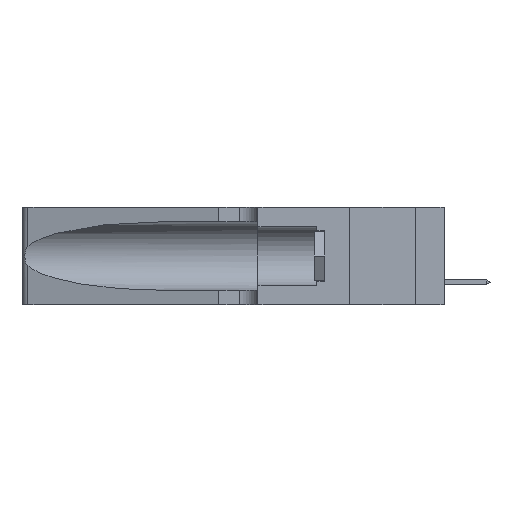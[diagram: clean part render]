
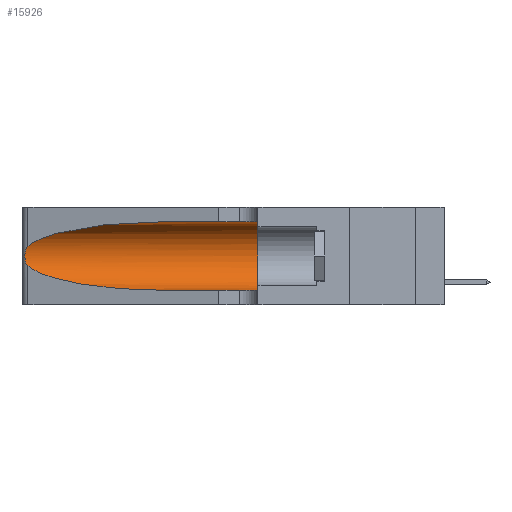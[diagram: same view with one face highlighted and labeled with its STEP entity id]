
A CAD part, left-side view. The second image highlights one B-rep face of the part: STEP entity #15926.
In plain terms, the highlighted cylindrical face has radius 3.308 mm (diameter 6.617 mm), a partial arc.
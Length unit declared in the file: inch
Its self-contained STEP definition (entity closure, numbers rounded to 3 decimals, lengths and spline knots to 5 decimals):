
#88 = CARTESIAN_POINT ( 'NONE',  ( 0.25487, 1.22718, 0.22369 ) ) ;
#142 = CARTESIAN_POINT ( 'NONE',  ( 0.25487, 1.22718, 0.22369 ) ) ;
#237 = CARTESIAN_POINT ( 'NONE',  ( 0.25854, 1.2359, 0.20912 ) ) ;
#312 = CARTESIAN_POINT ( 'NONE',  ( 0.25487, 1.22718, 0.22369 ) ) ;
#527 = CARTESIAN_POINT ( 'NONE',  ( 0.18966, 0.96281, 0.05475 ) ) ;
#576 = DIRECTION ( 'NONE',  ( 0., 0., -1. ) ) ;
#703 = VERTEX_POINT ( 'NONE', #16997 ) ;
#1011 = CARTESIAN_POINT ( 'NONE',  ( 0.1305, 0.35, 0.185 ) ) ;
#1067 = ORIENTED_EDGE ( 'NONE', *, *, #16218, .T. ) ;
#1242 = B_SPLINE_CURVE_WITH_KNOTS ( 'NONE', 3,
 ( #312, #6935, #6656, #5045, #237, #13346, #3399, #16834, #8630, #11989, #6796, #20068, #18690, #10314 ),
 .UNSPECIFIED., .F., .F.,
 ( 4, 2, 2, 2, 2, 2, 4 ),
 ( 0., 0.00027, 0.00053, 0.00107, 0.0016, 0.00187, 0.00214 ),
 .UNSPECIFIED. ) ;
#1402 = ORIENTED_EDGE ( 'NONE', *, *, #5150, .T. ) ;
#1642 = CARTESIAN_POINT ( 'NONE',  ( 0.2373, 1.15595, 0.28018 ) ) ;
#1899 = CARTESIAN_POINT ( 'NONE',  ( 0.25487, 1.22718, 0.14631 ) ) ;
#2563 = VECTOR ( 'NONE', #11613, 39.37008 ) ;
#3113 = CARTESIAN_POINT ( 'NONE',  ( 0.18966, 0.96281, 0.31525 ) ) ;
#3399 = CARTESIAN_POINT ( 'NONE',  ( 0.26075, 1.23896, 0.19203 ) ) ;
#4764 = VERTEX_POINT ( 'NONE', #5331 ) ;
#5045 = CARTESIAN_POINT ( 'NONE',  ( 0.25787, 1.23484, 0.2124 ) ) ;
#5150 = EDGE_CURVE ( 'NONE', #12302, #703, #18276, .T. ) ;
#5331 = CARTESIAN_POINT ( 'NONE',  ( 0.1305, 0.72297, 0.31525 ) ) ;
#5946 = EDGE_LOOP ( 'NONE', ( #1067, #15056, #21410, #1402, #20583, #12580 ) ) ;
#6241 = CARTESIAN_POINT ( 'NONE',  ( 0.1305, 0.72297, 0.31525 ) ) ;
#6656 = CARTESIAN_POINT ( 'NONE',  ( 0.25639, 1.23184, 0.21858 ) ) ;
#6796 = CARTESIAN_POINT ( 'NONE',  ( 0.25789, 1.23486, 0.15765 ) ) ;
#6935 = CARTESIAN_POINT ( 'NONE',  ( 0.25555, 1.22994, 0.2215 ) ) ;
#7349 = DIRECTION ( 'NONE',  ( 0., -1., 0. ) ) ;
#7574 = DIRECTION ( 'NONE',  ( 0., 1., 0. ) ) ;
#8630 = CARTESIAN_POINT ( 'NONE',  ( 0.26017, 1.23833, 0.17102 ) ) ;
#9499 = EDGE_CURVE ( 'NONE', #4764, #20645, #19708, .T. ) ;
#10314 = CARTESIAN_POINT ( 'NONE',  ( 0.25487, 1.22718, 0.14631 ) ) ;
#10537 = EDGE_CURVE ( 'NONE', #16110, #12302, #18402, .T. ) ;
#11613 = DIRECTION ( 'NONE',  ( 0., -1., 0. ) ) ;
#11989 = CARTESIAN_POINT ( 'NONE',  ( 0.25856, 1.23593, 0.16098 ) ) ;
#12199 = CARTESIAN_POINT ( 'NONE',  ( 0.1305, 0.72297, 0.05475 ) ) ;
#12302 = VERTEX_POINT ( 'NONE', #18582 ) ;
#12580 = ORIENTED_EDGE ( 'NONE', *, *, #9499, .F. ) ;
#12728 = CYLINDRICAL_SURFACE ( 'NONE', #15548, 0.13025 ) ;
#13346 = CARTESIAN_POINT ( 'NONE',  ( 0.26018, 1.23835, 0.19895 ) ) ;
#13550 = VERTEX_POINT ( 'NONE', #142 ) ;
#13698 = CARTESIAN_POINT ( 'NONE',  ( 0.2373, 1.15595, 0.08982 ) ) ;
#14036 = CARTESIAN_POINT ( 'NONE',  ( 0.1305, 0.35, 0.31525 ) ) ;
#14186 = CIRCLE ( 'NONE', #18389, 0.13025 ) ;
#14517 = EDGE_CURVE ( 'NONE', #13550, #16110, #1242, .T. ) ;
#15056 = ORIENTED_EDGE ( 'NONE', *, *, #14517, .T. ) ;
#15089 = FACE_OUTER_BOUND ( 'NONE', #5946, .T. ) ;
#15548 = AXIS2_PLACEMENT_3D ( 'NONE', #18931, #7349, #576 ) ;
#15926 = ADVANCED_FACE ( 'NONE', ( #15089 ), #12728, .F. ) ;
#15973 = CARTESIAN_POINT ( 'NONE',  ( 0.25487, 1.22718, 0.14631 ) ) ;
#16110 = VERTEX_POINT ( 'NONE', #15973 ) ;
#16218 = EDGE_CURVE ( 'NONE', #4764, #13550, #16390, .T. ) ;
#16390 =( BOUNDED_CURVE ( )  B_SPLINE_CURVE ( 3, ( #6241, #3113, #1642, #88 ),
 .UNSPECIFIED., .F., .F. ) 
 B_SPLINE_CURVE_WITH_KNOTS ( ( 4, 4 ),
 ( 1.5708, 2.84003 ),
 .UNSPECIFIED. ) 
 CURVE ( )  GEOMETRIC_REPRESENTATION_ITEM ( )  RATIONAL_B_SPLINE_CURVE ( ( 1., 0.87, 0.87, 1. ) ) 
 REPRESENTATION_ITEM ( '' )  );
#16834 = CARTESIAN_POINT ( 'NONE',  ( 0.26075, 1.23896, 0.178 ) ) ;
#16997 = CARTESIAN_POINT ( 'NONE',  ( 0.1305, 0.35, 0.05475 ) ) ;
#17157 = DIRECTION ( 'NONE',  ( 0., -1., 0. ) ) ;
#17594 = CARTESIAN_POINT ( 'NONE',  ( 0.1305, 1.61858, 0.31525 ) ) ;
#17614 = DIRECTION ( 'NONE',  ( 0., 0., 1. ) ) ;
#17772 = EDGE_CURVE ( 'NONE', #20645, #703, #14186, .T. ) ;
#18155 = CARTESIAN_POINT ( 'NONE',  ( 0.1305, 1.61858, 0.05475 ) ) ;
#18276 = LINE ( 'NONE', #18155, #2563 ) ;
#18389 = AXIS2_PLACEMENT_3D ( 'NONE', #1011, #7574, #17614 ) ;
#18402 =( BOUNDED_CURVE ( )  B_SPLINE_CURVE ( 3, ( #1899, #13698, #527, #12199 ),
 .UNSPECIFIED., .F., .F. ) 
 B_SPLINE_CURVE_WITH_KNOTS ( ( 4, 4 ),
 ( 3.44316, 4.71239 ),
 .UNSPECIFIED. ) 
 CURVE ( )  GEOMETRIC_REPRESENTATION_ITEM ( )  RATIONAL_B_SPLINE_CURVE ( ( 1., 0.87, 0.87, 1. ) ) 
 REPRESENTATION_ITEM ( '' )  );
#18582 = CARTESIAN_POINT ( 'NONE',  ( 0.1305, 0.72297, 0.05475 ) ) ;
#18690 = CARTESIAN_POINT ( 'NONE',  ( 0.25555, 1.22993, 0.14849 ) ) ;
#18931 = CARTESIAN_POINT ( 'NONE',  ( 0.1305, 1.61858, 0.185 ) ) ;
#19183 = VECTOR ( 'NONE', #17157, 39.37008 ) ;
#19708 = LINE ( 'NONE', #17594, #19183 ) ;
#20068 = CARTESIAN_POINT ( 'NONE',  ( 0.25639, 1.23186, 0.15144 ) ) ;
#20583 = ORIENTED_EDGE ( 'NONE', *, *, #17772, .F. ) ;
#20645 = VERTEX_POINT ( 'NONE', #14036 ) ;
#21410 = ORIENTED_EDGE ( 'NONE', *, *, #10537, .T. ) ;
